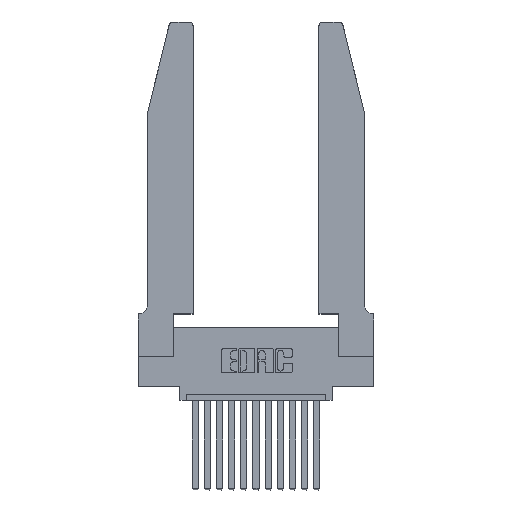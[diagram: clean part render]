
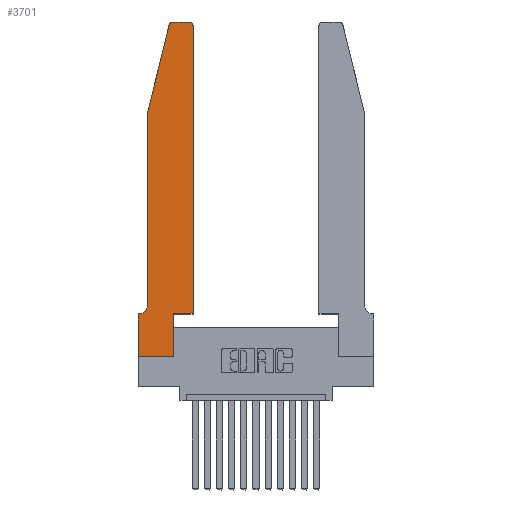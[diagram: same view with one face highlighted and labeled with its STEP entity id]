
A CAD part, top view. The second image highlights one B-rep face of the part: STEP entity #3701.
In plain terms, the highlighted planar face has unit normal (0, 0, 1).
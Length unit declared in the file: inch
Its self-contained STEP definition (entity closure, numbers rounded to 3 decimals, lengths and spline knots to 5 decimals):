
#624 = DIRECTION ( 'NONE',  ( 1., 0., 0. ) ) ;
#977 = DIRECTION ( 'NONE',  ( 0., -1., 0. ) ) ;
#1548 = CARTESIAN_POINT ( 'NONE',  ( 0.4505, 0.35, 0.37 ) ) ;
#1593 = VERTEX_POINT ( 'NONE', #5350 ) ;
#1717 = ORIENTED_EDGE ( 'NONE', *, *, #16972, .T. ) ;
#1786 = VERTEX_POINT ( 'NONE', #2959 ) ;
#1888 = VECTOR ( 'NONE', #15307, 39.37008 ) ;
#1908 = CIRCLE ( 'NONE', #15697, 0.07 ) ;
#2316 = CARTESIAN_POINT ( 'NONE',  ( 0.4505, 0.35, 0.37 ) ) ;
#2745 = VECTOR ( 'NONE', #5372, 39.37008 ) ;
#2750 = EDGE_CURVE ( 'NONE', #14027, #6830, #9486, .T. ) ;
#2810 = CARTESIAN_POINT ( 'NONE',  ( 0.0755, 2., 0.37 ) ) ;
#2959 = CARTESIAN_POINT ( 'NONE',  ( 0.4505, 2.72, 0.37 ) ) ;
#3101 = CARTESIAN_POINT ( 'NONE',  ( 0., 0.35, 0.37 ) ) ;
#3105 = VECTOR ( 'NONE', #5102, 39.37008 ) ;
#3212 = DIRECTION ( 'NONE',  ( -1., 0., 0. ) ) ;
#3289 = CARTESIAN_POINT ( 'NONE',  ( 0.4505, 0.35, 0.37 ) ) ;
#3344 = VECTOR ( 'NONE', #977, 39.37008 ) ;
#3369 = ORIENTED_EDGE ( 'NONE', *, *, #2750, .T. ) ;
#3385 = CARTESIAN_POINT ( 'NONE',  ( 0., 0., 0.37 ) ) ;
#3421 = ORIENTED_EDGE ( 'NONE', *, *, #7513, .T. ) ;
#3701 = ADVANCED_FACE ( 'NONE', ( #6334 ), #8560, .T. ) ;
#4004 = CARTESIAN_POINT ( 'NONE',  ( 0.2865, 0., 0.37 ) ) ;
#4028 = DIRECTION ( 'NONE',  ( 0., 0., 1. ) ) ;
#4598 = LINE ( 'NONE', #11878, #11249 ) ;
#4813 = CARTESIAN_POINT ( 'NONE',  ( 0.2865, 0.35, 0.37 ) ) ;
#4814 = LINE ( 'NONE', #1548, #13104 ) ;
#4887 = CIRCLE ( 'NONE', #5406, 0.03 ) ;
#4928 = CARTESIAN_POINT ( 'NONE',  ( 0.0755, 2., 0.37 ) ) ;
#5091 = DIRECTION ( 'NONE',  ( 1., 0., 0. ) ) ;
#5092 = ORIENTED_EDGE ( 'NONE', *, *, #6382, .T. ) ;
#5102 = DIRECTION ( 'NONE',  ( 0., 1., 0. ) ) ;
#5226 = CARTESIAN_POINT ( 'NONE',  ( 0.4205, 2.75, 0.37 ) ) ;
#5277 = EDGE_CURVE ( 'NONE', #1593, #14027, #12541, .T. ) ;
#5350 = CARTESIAN_POINT ( 'NONE',  ( 0., 0., 0.37 ) ) ;
#5356 = DIRECTION ( 'NONE',  ( 0., 1., 0. ) ) ;
#5372 = DIRECTION ( 'NONE',  ( -1., 0., 0. ) ) ;
#5406 = AXIS2_PLACEMENT_3D ( 'NONE', #11387, #11445, #10277 ) ;
#5556 = DIRECTION ( 'NONE',  ( -1., 0., 0. ) ) ;
#5972 = CIRCLE ( 'NONE', #9114, 0.03 ) ;
#6166 = VERTEX_POINT ( 'NONE', #15608 ) ;
#6334 = FACE_OUTER_BOUND ( 'NONE', #12877, .T. ) ;
#6346 = CARTESIAN_POINT ( 'NONE',  ( 0., 0., 0.37 ) ) ;
#6382 = EDGE_CURVE ( 'NONE', #9072, #1786, #4814, .T. ) ;
#6506 = ORIENTED_EDGE ( 'NONE', *, *, #13337, .T. ) ;
#6543 = DIRECTION ( 'NONE',  ( 1., 0., 0. ) ) ;
#6607 = LINE ( 'NONE', #11093, #16966 ) ;
#6781 = ORIENTED_EDGE ( 'NONE', *, *, #12592, .T. ) ;
#6830 = VERTEX_POINT ( 'NONE', #4813 ) ;
#7136 = VECTOR ( 'NONE', #5091, 39.37008 ) ;
#7194 = EDGE_CURVE ( 'NONE', #10186, #10667, #15387, .T. ) ;
#7360 = CARTESIAN_POINT ( 'NONE',  ( 0.25487, 2.72718, 0.37 ) ) ;
#7513 = EDGE_CURVE ( 'NONE', #16038, #6166, #13266, .T. ) ;
#7750 = EDGE_CURVE ( 'NONE', #6166, #10186, #1908, .T. ) ;
#7964 = EDGE_CURVE ( 'NONE', #17153, #14139, #6607, .T. ) ;
#8074 = EDGE_CURVE ( 'NONE', #10667, #1593, #13249, .T. ) ;
#8560 = PLANE ( 'NONE',  #10091 ) ;
#8819 = CARTESIAN_POINT ( 'NONE',  ( 0.2865, 0.35, 0.37 ) ) ;
#8889 = CARTESIAN_POINT ( 'NONE',  ( 0., 0.35, 0.37 ) ) ;
#9072 = VERTEX_POINT ( 'NONE', #3289 ) ;
#9114 = AXIS2_PLACEMENT_3D ( 'NONE', #11942, #4028, #6543 ) ;
#9486 = LINE ( 'NONE', #8819, #3105 ) ;
#10091 = AXIS2_PLACEMENT_3D ( 'NONE', #8889, #13005, #624 ) ;
#10186 = VERTEX_POINT ( 'NONE', #14562 ) ;
#10277 = DIRECTION ( 'NONE',  ( 1., 0., 0. ) ) ;
#10667 = VERTEX_POINT ( 'NONE', #3101 ) ;
#11093 = CARTESIAN_POINT ( 'NONE',  ( 0.2605, 2.75, 0.37 ) ) ;
#11249 = VECTOR ( 'NONE', #12224, 39.37008 ) ;
#11347 = EDGE_CURVE ( 'NONE', #11860, #16038, #4598, .T. ) ;
#11387 = CARTESIAN_POINT ( 'NONE',  ( 0.284, 2.72, 0.37 ) ) ;
#11445 = DIRECTION ( 'NONE',  ( 0., 0., 1. ) ) ;
#11532 = ORIENTED_EDGE ( 'NONE', *, *, #8074, .T. ) ;
#11860 = VERTEX_POINT ( 'NONE', #7360 ) ;
#11878 = CARTESIAN_POINT ( 'NONE',  ( 0.0755, 2., 0.37 ) ) ;
#11942 = CARTESIAN_POINT ( 'NONE',  ( 0.4205, 2.72, 0.37 ) ) ;
#11993 = VECTOR ( 'NONE', #12938, 39.37008 ) ;
#12224 = DIRECTION ( 'NONE',  ( -0.239, -0.971, 0. ) ) ;
#12379 = CARTESIAN_POINT ( 'NONE',  ( 0.284, 2.75, 0.37 ) ) ;
#12541 = LINE ( 'NONE', #6346, #7136 ) ;
#12592 = EDGE_CURVE ( 'NONE', #6830, #9072, #16772, .T. ) ;
#12877 = EDGE_LOOP ( 'NONE', ( #16253, #1717, #15819, #3421, #14663, #16728, #11532, #14456, #3369, #6781, #5092, #6506 ) ) ;
#12938 = DIRECTION ( 'NONE',  ( 1., 0., 0. ) ) ;
#13005 = DIRECTION ( 'NONE',  ( 0., 0., 1. ) ) ;
#13104 = VECTOR ( 'NONE', #5356, 39.37008 ) ;
#13249 = LINE ( 'NONE', #3385, #1888 ) ;
#13266 = LINE ( 'NONE', #4928, #3344 ) ;
#13323 = CARTESIAN_POINT ( 'NONE',  ( 0.0755, 0.35, 0.37 ) ) ;
#13337 = EDGE_CURVE ( 'NONE', #1786, #17153, #5972, .T. ) ;
#13522 = CARTESIAN_POINT ( 'NONE',  ( 0.0055, 0.42, 0.37 ) ) ;
#14027 = VERTEX_POINT ( 'NONE', #4004 ) ;
#14139 = VERTEX_POINT ( 'NONE', #12379 ) ;
#14456 = ORIENTED_EDGE ( 'NONE', *, *, #5277, .T. ) ;
#14562 = CARTESIAN_POINT ( 'NONE',  ( 0.0055, 0.35, 0.37 ) ) ;
#14663 = ORIENTED_EDGE ( 'NONE', *, *, #7750, .T. ) ;
#15307 = DIRECTION ( 'NONE',  ( 0., -1., 0. ) ) ;
#15387 = LINE ( 'NONE', #13323, #2745 ) ;
#15608 = CARTESIAN_POINT ( 'NONE',  ( 0.0755, 0.42, 0.37 ) ) ;
#15697 = AXIS2_PLACEMENT_3D ( 'NONE', #13522, #16127, #5556 ) ;
#15819 = ORIENTED_EDGE ( 'NONE', *, *, #11347, .T. ) ;
#16038 = VERTEX_POINT ( 'NONE', #2810 ) ;
#16127 = DIRECTION ( 'NONE',  ( 0., 0., -1. ) ) ;
#16253 = ORIENTED_EDGE ( 'NONE', *, *, #7964, .T. ) ;
#16728 = ORIENTED_EDGE ( 'NONE', *, *, #7194, .T. ) ;
#16772 = LINE ( 'NONE', #2316, #11993 ) ;
#16966 = VECTOR ( 'NONE', #3212, 39.37008 ) ;
#16972 = EDGE_CURVE ( 'NONE', #14139, #11860, #4887, .T. ) ;
#17153 = VERTEX_POINT ( 'NONE', #5226 ) ;
